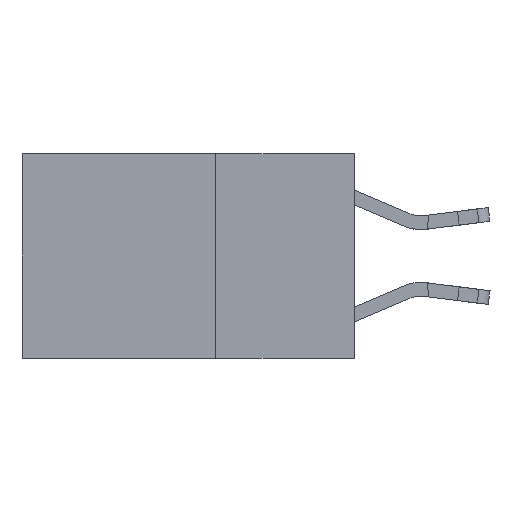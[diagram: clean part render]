
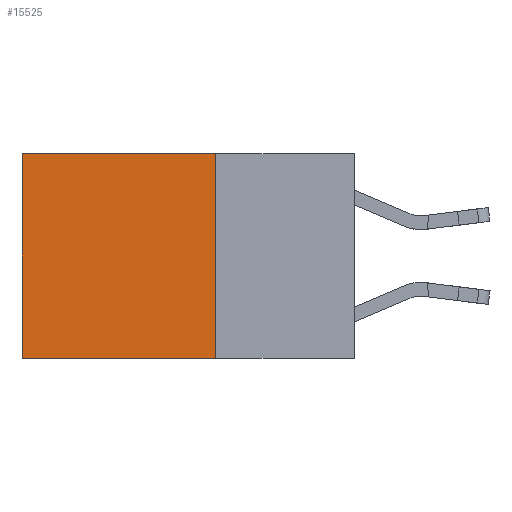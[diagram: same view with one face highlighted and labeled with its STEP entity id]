
A CAD part, left-side view. The second image highlights one B-rep face of the part: STEP entity #15525.
In plain terms, the highlighted planar face has unit normal (-1, 0, 0).
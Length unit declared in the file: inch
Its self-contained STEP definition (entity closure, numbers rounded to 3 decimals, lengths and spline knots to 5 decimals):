
#598 = CARTESIAN_POINT ( 'NONE',  ( 0.2625, 0.25, 0. ) ) ;
#892 = LINE ( 'NONE', #598, #9911 ) ;
#1526 = ORIENTED_EDGE ( 'NONE', *, *, #18948, .F. ) ;
#2079 = CARTESIAN_POINT ( 'NONE',  ( 0.2625, 0.25, -0.37 ) ) ;
#2225 = DIRECTION ( 'NONE',  ( 1., 0., 0. ) ) ;
#3589 = ORIENTED_EDGE ( 'NONE', *, *, #16785, .T. ) ;
#3958 = DIRECTION ( 'NONE',  ( 0., 0., -1. ) ) ;
#5025 = AXIS2_PLACEMENT_3D ( 'NONE', #5183, #2225, #9689 ) ;
#5183 = CARTESIAN_POINT ( 'NONE',  ( 0.2625, 0.25, 0. ) ) ;
#6145 = DIRECTION ( 'NONE',  ( 0., 1., 0. ) ) ;
#6276 = CARTESIAN_POINT ( 'NONE',  ( 0.2625, 0.25, 0. ) ) ;
#7098 = FACE_OUTER_BOUND ( 'NONE', #7749, .T. ) ;
#7707 = VECTOR ( 'NONE', #13993, 39.37008 ) ;
#7749 = EDGE_LOOP ( 'NONE', ( #3589, #15337, #1526, #10950 ) ) ;
#9403 = DIRECTION ( 'NONE',  ( 0., 1., 0. ) ) ;
#9419 = VECTOR ( 'NONE', #3958, 39.37008 ) ;
#9689 = DIRECTION ( 'NONE',  ( 0., 0., -1. ) ) ;
#9911 = VECTOR ( 'NONE', #9403, 39.37008 ) ;
#10049 = LINE ( 'NONE', #17150, #7707 ) ;
#10570 = VERTEX_POINT ( 'NONE', #2079 ) ;
#10793 = LINE ( 'NONE', #15701, #9419 ) ;
#10950 = ORIENTED_EDGE ( 'NONE', *, *, #14823, .T. ) ;
#11252 = CARTESIAN_POINT ( 'NONE',  ( 0.2625, 0.6, 0. ) ) ;
#12212 = VERTEX_POINT ( 'NONE', #6276 ) ;
#12230 = EDGE_CURVE ( 'NONE', #10570, #16146, #14632, .T. ) ;
#13044 = VECTOR ( 'NONE', #6145, 39.37008 ) ;
#13421 = CARTESIAN_POINT ( 'NONE',  ( 0.2625, 0.25, -0.37 ) ) ;
#13991 = VERTEX_POINT ( 'NONE', #11252 ) ;
#13993 = DIRECTION ( 'NONE',  ( 0., 0., -1. ) ) ;
#14632 = LINE ( 'NONE', #13421, #13044 ) ;
#14823 = EDGE_CURVE ( 'NONE', #12212, #13991, #892, .T. ) ;
#15337 = ORIENTED_EDGE ( 'NONE', *, *, #12230, .F. ) ;
#15411 = PLANE ( 'NONE',  #5025 ) ;
#15525 = ADVANCED_FACE ( 'NONE', ( #7098 ), #15411, .F. ) ;
#15701 = CARTESIAN_POINT ( 'NONE',  ( 0.2625, 0.6, 0. ) ) ;
#16146 = VERTEX_POINT ( 'NONE', #16622 ) ;
#16622 = CARTESIAN_POINT ( 'NONE',  ( 0.2625, 0.6, -0.37 ) ) ;
#16785 = EDGE_CURVE ( 'NONE', #13991, #16146, #10793, .T. ) ;
#17150 = CARTESIAN_POINT ( 'NONE',  ( 0.2625, 0.25, 0. ) ) ;
#18948 = EDGE_CURVE ( 'NONE', #12212, #10570, #10049, .T. ) ;
